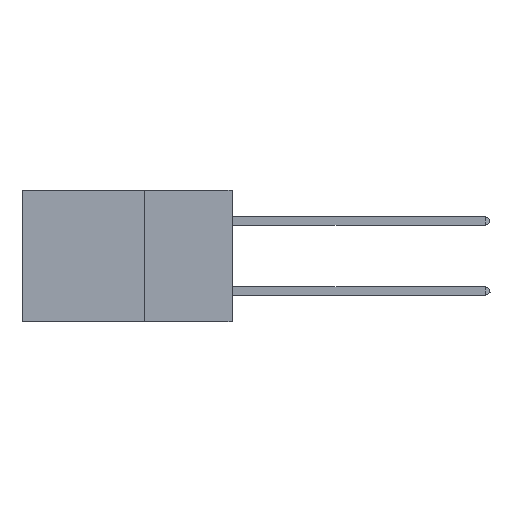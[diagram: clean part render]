
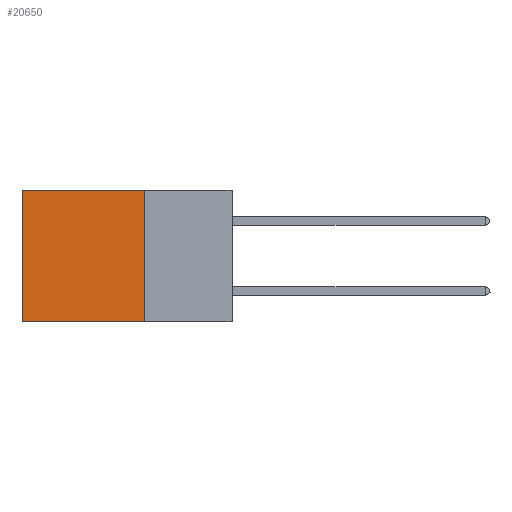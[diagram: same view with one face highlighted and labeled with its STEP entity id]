
A CAD part, left-side view. The second image highlights one B-rep face of the part: STEP entity #20650.
In plain terms, the highlighted planar face has unit normal (-1, 0, 0).
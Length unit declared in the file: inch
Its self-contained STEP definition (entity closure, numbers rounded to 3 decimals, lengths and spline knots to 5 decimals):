
#700 = CARTESIAN_POINT ( 'NONE',  ( 0.2875, 0.6, 0. ) ) ;
#809 = ORIENTED_EDGE ( 'NONE', *, *, #17126, .F. ) ;
#845 = VECTOR ( 'NONE', #8893, 39.37008 ) ;
#1038 = CARTESIAN_POINT ( 'NONE',  ( 0.2875, 0.25, -0.375 ) ) ;
#1468 = DIRECTION ( 'NONE',  ( 0., 0., -1. ) ) ;
#1551 = LINE ( 'NONE', #7886, #14452 ) ;
#3847 = ORIENTED_EDGE ( 'NONE', *, *, #13918, .T. ) ;
#5471 = DIRECTION ( 'NONE',  ( 0., 0., -1. ) ) ;
#6078 = FACE_OUTER_BOUND ( 'NONE', #15053, .T. ) ;
#6713 = VERTEX_POINT ( 'NONE', #7131 ) ;
#7131 = CARTESIAN_POINT ( 'NONE',  ( 0.2875, 0.6, -0.375 ) ) ;
#7886 = CARTESIAN_POINT ( 'NONE',  ( 0.2875, 0.25, -0.375 ) ) ;
#8131 = CARTESIAN_POINT ( 'NONE',  ( 0.2875, 0.25, -0.375 ) ) ;
#8480 = AXIS2_PLACEMENT_3D ( 'NONE', #1038, #9716, #1468 ) ;
#8702 = EDGE_CURVE ( 'NONE', #14537, #6713, #1551, .T. ) ;
#8893 = DIRECTION ( 'NONE',  ( 0., 0., -1. ) ) ;
#9488 = LINE ( 'NONE', #14085, #17886 ) ;
#9689 = LINE ( 'NONE', #15549, #14953 ) ;
#9716 = DIRECTION ( 'NONE',  ( 1., 0., 0. ) ) ;
#10116 = ORIENTED_EDGE ( 'NONE', *, *, #21371, .T. ) ;
#10511 = CARTESIAN_POINT ( 'NONE',  ( 0.2875, 0.25, -0.375 ) ) ;
#11463 = VERTEX_POINT ( 'NONE', #19363 ) ;
#13918 = EDGE_CURVE ( 'NONE', #15487, #6713, #9689, .T. ) ;
#14085 = CARTESIAN_POINT ( 'NONE',  ( 0.2875, 0.25, 0. ) ) ;
#14452 = VECTOR ( 'NONE', #14595, 39.37008 ) ;
#14537 = VERTEX_POINT ( 'NONE', #8131 ) ;
#14595 = DIRECTION ( 'NONE',  ( 0., 1., 0. ) ) ;
#14953 = VECTOR ( 'NONE', #5471, 39.37008 ) ;
#15053 = EDGE_LOOP ( 'NONE', ( #3847, #21212, #809, #10116 ) ) ;
#15487 = VERTEX_POINT ( 'NONE', #700 ) ;
#15549 = CARTESIAN_POINT ( 'NONE',  ( 0.2875, 0.6, -0.375 ) ) ;
#17126 = EDGE_CURVE ( 'NONE', #11463, #14537, #19223, .T. ) ;
#17431 = DIRECTION ( 'NONE',  ( 0., 1., 0. ) ) ;
#17782 = PLANE ( 'NONE',  #8480 ) ;
#17886 = VECTOR ( 'NONE', #17431, 39.37008 ) ;
#19223 = LINE ( 'NONE', #10511, #845 ) ;
#19363 = CARTESIAN_POINT ( 'NONE',  ( 0.2875, 0.25, 0. ) ) ;
#20650 = ADVANCED_FACE ( 'NONE', ( #6078 ), #17782, .F. ) ;
#21212 = ORIENTED_EDGE ( 'NONE', *, *, #8702, .F. ) ;
#21371 = EDGE_CURVE ( 'NONE', #11463, #15487, #9488, .T. ) ;
